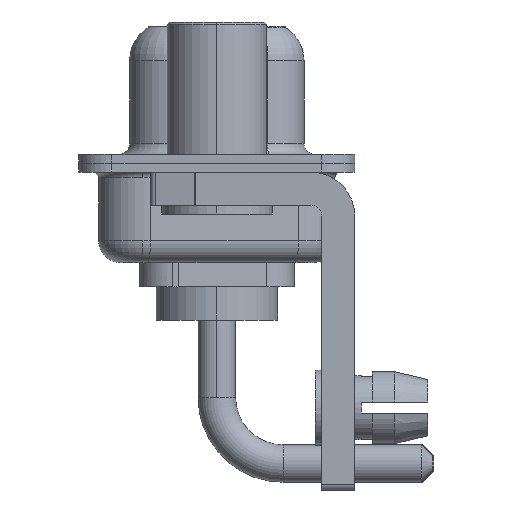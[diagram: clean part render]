
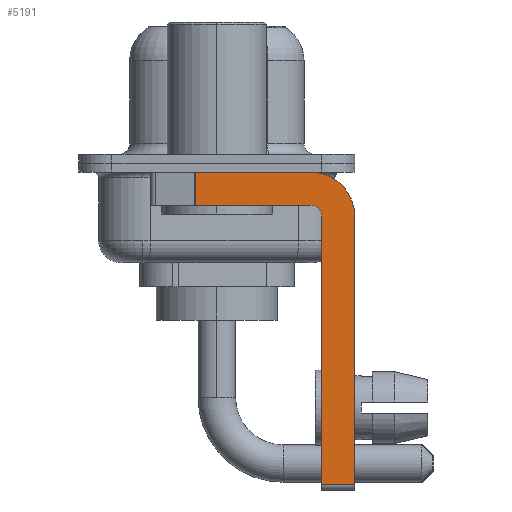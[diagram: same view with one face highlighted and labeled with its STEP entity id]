
A CAD part, left-side view. The second image highlights one B-rep face of the part: STEP entity #5191.
In plain terms, the highlighted planar face has unit normal (-1, 0, 0).
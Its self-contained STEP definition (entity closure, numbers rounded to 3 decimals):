
#221 = ORIENTED_EDGE ( 'NONE', *, *, #12832, .T. ) ;
#445 = ORIENTED_EDGE ( 'NONE', *, *, #3171, .T. ) ;
#840 = CARTESIAN_POINT ( 'NONE',  ( -2.9, -6.25, -2.4 ) ) ;
#933 = DIRECTION ( 'NONE',  ( 0., 0., 1. ) ) ;
#1374 = LINE ( 'NONE', #5428, #13297 ) ;
#1443 = EDGE_CURVE ( 'NONE', #8438, #2971, #11218, .T. ) ;
#1503 = EDGE_LOOP ( 'NONE', ( #3449, #445, #6694, #16158, #4383, #221, #12485, #9591 ) ) ;
#1589 = DIRECTION ( 'NONE',  ( 0., -1., 0. ) ) ;
#1615 = CARTESIAN_POINT ( 'NONE',  ( -2.9, -6.25, -2.4 ) ) ;
#1688 = CARTESIAN_POINT ( 'NONE',  ( -2.9, -4.75, -14.55 ) ) ;
#1735 = DIRECTION ( 'NONE',  ( 0., 0., -1. ) ) ;
#2168 = AXIS2_PLACEMENT_3D ( 'NONE', #15072, #9524, #9437 ) ;
#2971 = VERTEX_POINT ( 'NONE', #17056 ) ;
#3055 = PLANE ( 'NONE',  #16258 ) ;
#3102 = DIRECTION ( 'NONE',  ( 0., 0., -1. ) ) ;
#3171 = EDGE_CURVE ( 'NONE', #14812, #8772, #5794, .T. ) ;
#3449 = ORIENTED_EDGE ( 'NONE', *, *, #3574, .F. ) ;
#3574 = EDGE_CURVE ( 'NONE', #14812, #11864, #1374, .T. ) ;
#3978 = CARTESIAN_POINT ( 'NONE',  ( -2.9, 0.978, -1.9 ) ) ;
#4007 = VERTEX_POINT ( 'NONE', #1688 ) ;
#4145 = DIRECTION ( 'NONE',  ( 0., 0., -1. ) ) ;
#4383 = ORIENTED_EDGE ( 'NONE', *, *, #10492, .F. ) ;
#4450 = VERTEX_POINT ( 'NONE', #12395 ) ;
#4564 = EDGE_CURVE ( 'NONE', #11864, #14988, #7326, .T. ) ;
#5053 = CARTESIAN_POINT ( 'NONE',  ( -2.9, -4.25, -14.55 ) ) ;
#5090 = VECTOR ( 'NONE', #4145, 1000. ) ;
#5191 = ADVANCED_FACE ( 'NONE', ( #7046 ), #3055, .F. ) ;
#5265 = CARTESIAN_POINT ( 'NONE',  ( -2.9, -4.25, -0.4 ) ) ;
#5428 = CARTESIAN_POINT ( 'NONE',  ( -2.9, 3., -0.4 ) ) ;
#5530 = VECTOR ( 'NONE', #3102, 1000. ) ;
#5794 = LINE ( 'NONE', #3978, #5090 ) ;
#6034 = CARTESIAN_POINT ( 'NONE',  ( -2.9, 0.978, -0.4 ) ) ;
#6694 = ORIENTED_EDGE ( 'NONE', *, *, #6978, .F. ) ;
#6978 = EDGE_CURVE ( 'NONE', #2971, #8772, #9913, .T. ) ;
#7046 = FACE_OUTER_BOUND ( 'NONE', #1503, .T. ) ;
#7326 = CIRCLE ( 'NONE', #9596, 2. ) ;
#7834 = DIRECTION ( 'NONE',  ( 0., 1., 0. ) ) ;
#8319 = CARTESIAN_POINT ( 'NONE',  ( -2.9, -4.75, -2.4 ) ) ;
#8438 = VERTEX_POINT ( 'NONE', #8319 ) ;
#8478 = CARTESIAN_POINT ( 'NONE',  ( -2.9, -4.25, -2.4 ) ) ;
#8772 = VERTEX_POINT ( 'NONE', #10785 ) ;
#9437 = DIRECTION ( 'NONE',  ( 0., 0., 1. ) ) ;
#9524 = DIRECTION ( 'NONE',  ( -1., 0., 0. ) ) ;
#9591 = ORIENTED_EDGE ( 'NONE', *, *, #4564, .F. ) ;
#9596 = AXIS2_PLACEMENT_3D ( 'NONE', #9916, #10085, #16864 ) ;
#9715 = VECTOR ( 'NONE', #933, 1000. ) ;
#9913 = LINE ( 'NONE', #10832, #10808 ) ;
#9916 = CARTESIAN_POINT ( 'NONE',  ( -2.9, -4.25, -2.4 ) ) ;
#10085 = DIRECTION ( 'NONE',  ( 1., 0., 0. ) ) ;
#10492 = EDGE_CURVE ( 'NONE', #4007, #8438, #13043, .T. ) ;
#10785 = CARTESIAN_POINT ( 'NONE',  ( -2.9, 0.978, -1.9 ) ) ;
#10808 = VECTOR ( 'NONE', #7834, 1000. ) ;
#10832 = CARTESIAN_POINT ( 'NONE',  ( -2.9, -4.25, -1.9 ) ) ;
#11086 = LINE ( 'NONE', #1615, #5530 ) ;
#11188 = VECTOR ( 'NONE', #1589, 1000. ) ;
#11218 = CIRCLE ( 'NONE', #2168, 0.5 ) ;
#11864 = VERTEX_POINT ( 'NONE', #5265 ) ;
#12395 = CARTESIAN_POINT ( 'NONE',  ( -2.9, -6.25, -14.55 ) ) ;
#12437 = DIRECTION ( 'NONE',  ( 0., -1., 0. ) ) ;
#12460 = EDGE_CURVE ( 'NONE', #14988, #4450, #11086, .T. ) ;
#12485 = ORIENTED_EDGE ( 'NONE', *, *, #12460, .F. ) ;
#12832 = EDGE_CURVE ( 'NONE', #4007, #4450, #17155, .T. ) ;
#12963 = CARTESIAN_POINT ( 'NONE',  ( -2.9, -4.75, -14.8 ) ) ;
#13043 = LINE ( 'NONE', #12963, #9715 ) ;
#13297 = VECTOR ( 'NONE', #12437, 1000. ) ;
#13857 = DIRECTION ( 'NONE',  ( 1., 0., 0. ) ) ;
#14812 = VERTEX_POINT ( 'NONE', #6034 ) ;
#14988 = VERTEX_POINT ( 'NONE', #840 ) ;
#15072 = CARTESIAN_POINT ( 'NONE',  ( -2.9, -4.25, -2.4 ) ) ;
#16158 = ORIENTED_EDGE ( 'NONE', *, *, #1443, .F. ) ;
#16258 = AXIS2_PLACEMENT_3D ( 'NONE', #8478, #13857, #1735 ) ;
#16864 = DIRECTION ( 'NONE',  ( 0., 0., -1. ) ) ;
#17056 = CARTESIAN_POINT ( 'NONE',  ( -2.9, -4.25, -1.9 ) ) ;
#17155 = LINE ( 'NONE', #5053, #11188 ) ;
